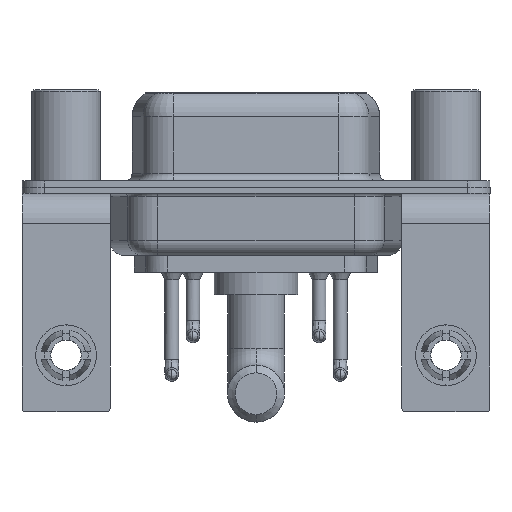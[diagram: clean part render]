
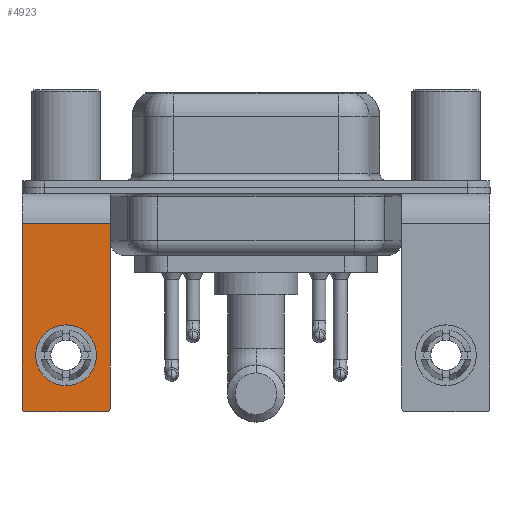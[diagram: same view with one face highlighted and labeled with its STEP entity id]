
A CAD part, front view. The second image highlights one B-rep face of the part: STEP entity #4923.
In plain terms, the highlighted planar face has unit normal (0, -1, 0).
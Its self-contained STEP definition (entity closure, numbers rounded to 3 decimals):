
#31 = AXIS2_PLACEMENT_3D ( 'NONE', #7892, #150, #10820 ) ;
#150 = DIRECTION ( 'NONE',  ( 0., -1., 0. ) ) ;
#592 = CARTESIAN_POINT ( 'NONE',  ( -2.65, -6.25, -14.8 ) ) ;
#875 = DIRECTION ( 'NONE',  ( 0., -1., 0. ) ) ;
#1305 = VERTEX_POINT ( 'NONE', #9320 ) ;
#1951 = CIRCLE ( 'NONE', #31, 0.25 ) ;
#2156 = ORIENTED_EDGE ( 'NONE', *, *, #3052, .T. ) ;
#2228 = AXIS2_PLACEMENT_3D ( 'NONE', #8689, #17838, #11722 ) ;
#2229 = ORIENTED_EDGE ( 'NONE', *, *, #14514, .T. ) ;
#2283 = AXIS2_PLACEMENT_3D ( 'NONE', #14877, #875, #11650 ) ;
#2298 = DIRECTION ( 'NONE',  ( 0., 0., 1. ) ) ;
#2662 = CARTESIAN_POINT ( 'NONE',  ( 2.65, -6.25, -14.8 ) ) ;
#3052 = EDGE_CURVE ( 'NONE', #1305, #12644, #9608, .T. ) ;
#3786 = EDGE_CURVE ( 'NONE', #11953, #4745, #18501, .T. ) ;
#3811 = PLANE ( 'NONE',  #13886 ) ;
#3885 = CIRCLE ( 'NONE', #2283, 0.25 ) ;
#3990 = CARTESIAN_POINT ( 'NONE',  ( -2.9, -6.25, -2.4 ) ) ;
#4608 = CARTESIAN_POINT ( 'NONE',  ( -2.9, -6.25, -14.55 ) ) ;
#4702 = CARTESIAN_POINT ( 'NONE',  ( 2.9, -6.25, -2.4 ) ) ;
#4745 = VERTEX_POINT ( 'NONE', #10757 ) ;
#4923 = ADVANCED_FACE ( 'NONE', ( #8221, #17571 ), #3811, .F. ) ;
#4982 = EDGE_LOOP ( 'NONE', ( #12878, #2229, #13579, #10042, #10172, #5048 ) ) ;
#5048 = ORIENTED_EDGE ( 'NONE', *, *, #3786, .T. ) ;
#5306 = ORIENTED_EDGE ( 'NONE', *, *, #11639, .T. ) ;
#5491 = DIRECTION ( 'NONE',  ( 0., 0., -1. ) ) ;
#5695 = LINE ( 'NONE', #3990, #19777 ) ;
#5739 = CARTESIAN_POINT ( 'NONE',  ( 2.9, -6.25, -2.4 ) ) ;
#5952 = EDGE_LOOP ( 'NONE', ( #2156, #5306 ) ) ;
#7043 = DIRECTION ( 'NONE',  ( -1., 0., 0. ) ) ;
#7802 = VERTEX_POINT ( 'NONE', #17204 ) ;
#7854 = DIRECTION ( 'NONE',  ( 0., 1., 0. ) ) ;
#7892 = CARTESIAN_POINT ( 'NONE',  ( -2.65, -6.25, -14.55 ) ) ;
#8049 = CARTESIAN_POINT ( 'NONE',  ( 2.9, -6.25, -2.4 ) ) ;
#8221 = FACE_BOUND ( 'NONE', #5952, .T. ) ;
#8423 = CARTESIAN_POINT ( 'NONE',  ( 2.9, -6.25, -2.4 ) ) ;
#8550 = VERTEX_POINT ( 'NONE', #4608 ) ;
#8652 = CARTESIAN_POINT ( 'NONE',  ( 2.9, -6.25, -14.8 ) ) ;
#8689 = CARTESIAN_POINT ( 'NONE',  ( 0., -6.25, -11.07 ) ) ;
#8901 = VERTEX_POINT ( 'NONE', #2662 ) ;
#9320 = CARTESIAN_POINT ( 'NONE',  ( 0., -6.25, -13.07 ) ) ;
#9608 = CIRCLE ( 'NONE', #2228, 2. ) ;
#9948 = DIRECTION ( 'NONE',  ( 0., 1., 0. ) ) ;
#10042 = ORIENTED_EDGE ( 'NONE', *, *, #16931, .T. ) ;
#10172 = ORIENTED_EDGE ( 'NONE', *, *, #14038, .F. ) ;
#10654 = DIRECTION ( 'NONE',  ( 0., 0., -1. ) ) ;
#10757 = CARTESIAN_POINT ( 'NONE',  ( -2.9, -6.25, -2.4 ) ) ;
#10820 = DIRECTION ( 'NONE',  ( 0., 0., 1. ) ) ;
#11214 = CIRCLE ( 'NONE', #12501, 2. ) ;
#11639 = EDGE_CURVE ( 'NONE', #12644, #1305, #11214, .T. ) ;
#11650 = DIRECTION ( 'NONE',  ( 0., 0., 1. ) ) ;
#11722 = DIRECTION ( 'NONE',  ( 0., 0., 1. ) ) ;
#11920 = EDGE_CURVE ( 'NONE', #8901, #12217, #17704, .T. ) ;
#11953 = VERTEX_POINT ( 'NONE', #5739 ) ;
#12217 = VERTEX_POINT ( 'NONE', #592 ) ;
#12501 = AXIS2_PLACEMENT_3D ( 'NONE', #17754, #7854, #14011 ) ;
#12644 = VERTEX_POINT ( 'NONE', #18470 ) ;
#12878 = ORIENTED_EDGE ( 'NONE', *, *, #19699, .T. ) ;
#13579 = ORIENTED_EDGE ( 'NONE', *, *, #11920, .F. ) ;
#13873 = LINE ( 'NONE', #4702, #15131 ) ;
#13886 = AXIS2_PLACEMENT_3D ( 'NONE', #8423, #9948, #2298 ) ;
#14011 = DIRECTION ( 'NONE',  ( 0., 0., 1. ) ) ;
#14038 = EDGE_CURVE ( 'NONE', #11953, #7802, #13873, .T. ) ;
#14218 = DIRECTION ( 'NONE',  ( -1., 0., 0. ) ) ;
#14514 = EDGE_CURVE ( 'NONE', #8550, #12217, #1951, .T. ) ;
#14877 = CARTESIAN_POINT ( 'NONE',  ( 2.65, -6.25, -14.55 ) ) ;
#15131 = VECTOR ( 'NONE', #10654, 1000. ) ;
#16293 = VECTOR ( 'NONE', #14218, 1000. ) ;
#16931 = EDGE_CURVE ( 'NONE', #8901, #7802, #3885, .T. ) ;
#17204 = CARTESIAN_POINT ( 'NONE',  ( 2.9, -6.25, -14.55 ) ) ;
#17571 = FACE_OUTER_BOUND ( 'NONE', #4982, .T. ) ;
#17704 = LINE ( 'NONE', #8652, #19550 ) ;
#17754 = CARTESIAN_POINT ( 'NONE',  ( 0., -6.25, -11.07 ) ) ;
#17838 = DIRECTION ( 'NONE',  ( 0., 1., 0. ) ) ;
#18470 = CARTESIAN_POINT ( 'NONE',  ( 0., -6.25, -9.07 ) ) ;
#18501 = LINE ( 'NONE', #8049, #16293 ) ;
#19550 = VECTOR ( 'NONE', #7043, 1000. ) ;
#19699 = EDGE_CURVE ( 'NONE', #4745, #8550, #5695, .T. ) ;
#19777 = VECTOR ( 'NONE', #5491, 1000. ) ;
